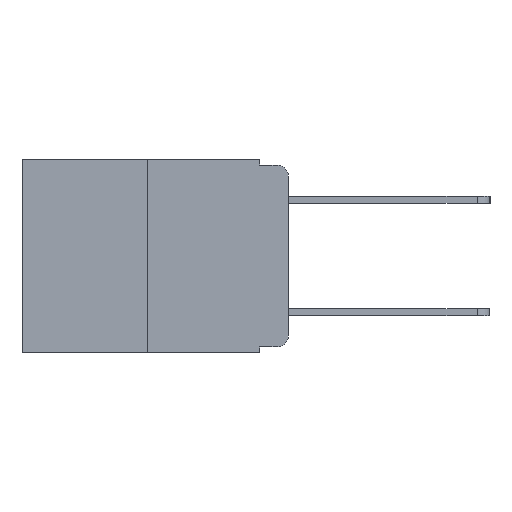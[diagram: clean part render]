
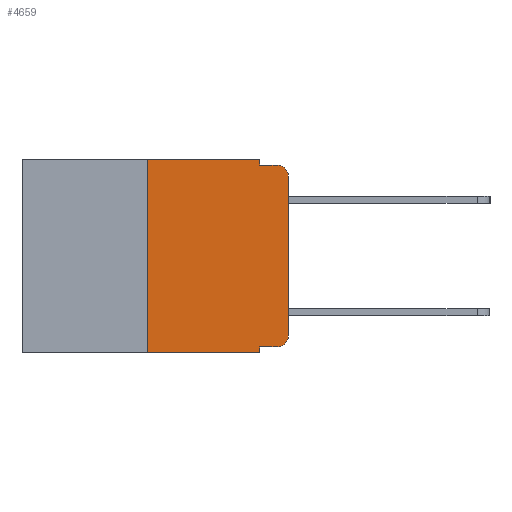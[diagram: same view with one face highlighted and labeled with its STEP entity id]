
A CAD part, left-side view. The second image highlights one B-rep face of the part: STEP entity #4659.
In plain terms, the highlighted planar face has unit normal (-1, 0, 0).
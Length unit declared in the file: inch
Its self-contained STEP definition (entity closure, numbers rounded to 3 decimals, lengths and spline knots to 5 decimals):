
#343 = DIRECTION ( 'NONE',  ( 0., 0., -1. ) ) ;
#415 = ORIENTED_EDGE ( 'NONE', *, *, #500, .T. ) ;
#500 = EDGE_CURVE ( 'NONE', #1813, #5621, #2623, .T. ) ;
#789 = LINE ( 'NONE', #902, #12038 ) ;
#824 = VERTEX_POINT ( 'NONE', #6479 ) ;
#839 = CARTESIAN_POINT ( 'NONE',  ( 0., 0.051, -0.343 ) ) ;
#902 = CARTESIAN_POINT ( 'NONE',  ( 0., 0.051, 0. ) ) ;
#933 = ORIENTED_EDGE ( 'NONE', *, *, #5554, .F. ) ;
#950 = VERTEX_POINT ( 'NONE', #839 ) ;
#1013 = VERTEX_POINT ( 'NONE', #8694 ) ;
#1298 = CARTESIAN_POINT ( 'NONE',  ( 0., 0.25, 0. ) ) ;
#1650 = VECTOR ( 'NONE', #11972, 39.37008 ) ;
#1764 = VERTEX_POINT ( 'NONE', #9532 ) ;
#1813 = VERTEX_POINT ( 'NONE', #7190 ) ;
#1817 = DIRECTION ( 'NONE',  ( 0., 0., -1. ) ) ;
#1917 = AXIS2_PLACEMENT_3D ( 'NONE', #5327, #12515, #6460 ) ;
#2474 = AXIS2_PLACEMENT_3D ( 'NONE', #7707, #5722, #5657 ) ;
#2623 = CIRCLE ( 'NONE', #3222, 0.02 ) ;
#2823 = CIRCLE ( 'NONE', #1917, 0.02 ) ;
#2984 = LINE ( 'NONE', #5390, #6049 ) ;
#3222 = AXIS2_PLACEMENT_3D ( 'NONE', #10448, #12787, #1817 ) ;
#3319 = VERTEX_POINT ( 'NONE', #11322 ) ;
#3447 = ORIENTED_EDGE ( 'NONE', *, *, #7054, .F. ) ;
#3523 = FACE_OUTER_BOUND ( 'NONE', #4366, .T. ) ;
#3734 = ORIENTED_EDGE ( 'NONE', *, *, #13476, .F. ) ;
#3756 = EDGE_CURVE ( 'NONE', #11343, #1813, #7503, .T. ) ;
#4064 = EDGE_CURVE ( 'NONE', #1013, #950, #789, .T. ) ;
#4366 = EDGE_LOOP ( 'NONE', ( #6656, #415, #3447, #933, #3734, #6722, #6639, #5891, #5738, #6790 ) ) ;
#4580 = CARTESIAN_POINT ( 'NONE',  ( 0., 0.473, -0.343 ) ) ;
#4587 = VECTOR ( 'NONE', #6284, 39.37008 ) ;
#4601 = DIRECTION ( 'NONE',  ( 0., -1., 0. ) ) ;
#4659 = ADVANCED_FACE ( 'NONE', ( #3523 ), #4942, .F. ) ;
#4846 = EDGE_CURVE ( 'NONE', #824, #12397, #6729, .T. ) ;
#4928 = EDGE_CURVE ( 'NONE', #824, #950, #10919, .T. ) ;
#4942 = PLANE ( 'NONE',  #2474 ) ;
#4946 = CARTESIAN_POINT ( 'NONE',  ( 0., 0., 0. ) ) ;
#5255 = CARTESIAN_POINT ( 'NONE',  ( 0., 0.02, -0.01 ) ) ;
#5327 = CARTESIAN_POINT ( 'NONE',  ( 0., 0.02, -0.313 ) ) ;
#5390 = CARTESIAN_POINT ( 'NONE',  ( 0., 0.051, -0.333 ) ) ;
#5554 = EDGE_CURVE ( 'NONE', #7035, #3319, #12079, .T. ) ;
#5621 = VERTEX_POINT ( 'NONE', #5255 ) ;
#5657 = DIRECTION ( 'NONE',  ( 0., 0., -1. ) ) ;
#5722 = DIRECTION ( 'NONE',  ( 1., 0., 0. ) ) ;
#5738 = ORIENTED_EDGE ( 'NONE', *, *, #13299, .T. ) ;
#5744 = CARTESIAN_POINT ( 'NONE',  ( 0., 0.051, 0. ) ) ;
#5773 = CARTESIAN_POINT ( 'NONE',  ( 0., 0.473, 0. ) ) ;
#5891 = ORIENTED_EDGE ( 'NONE', *, *, #4064, .F. ) ;
#6049 = VECTOR ( 'NONE', #11622, 39.37008 ) ;
#6055 = DIRECTION ( 'NONE',  ( 0., 0., 1. ) ) ;
#6284 = DIRECTION ( 'NONE',  ( 0., 0., 1. ) ) ;
#6460 = DIRECTION ( 'NONE',  ( 0., 0., -1. ) ) ;
#6479 = CARTESIAN_POINT ( 'NONE',  ( 0., 0.25, -0.343 ) ) ;
#6639 = ORIENTED_EDGE ( 'NONE', *, *, #4928, .T. ) ;
#6656 = ORIENTED_EDGE ( 'NONE', *, *, #3756, .T. ) ;
#6722 = ORIENTED_EDGE ( 'NONE', *, *, #4846, .F. ) ;
#6729 = LINE ( 'NONE', #9146, #12103 ) ;
#6790 = ORIENTED_EDGE ( 'NONE', *, *, #12036, .T. ) ;
#7035 = VERTEX_POINT ( 'NONE', #5744 ) ;
#7054 = EDGE_CURVE ( 'NONE', #3319, #5621, #10461, .T. ) ;
#7190 = CARTESIAN_POINT ( 'NONE',  ( 0., 0., -0.03 ) ) ;
#7503 = LINE ( 'NONE', #4946, #4587 ) ;
#7707 = CARTESIAN_POINT ( 'NONE',  ( 0., 0.473, 0. ) ) ;
#7772 = DIRECTION ( 'NONE',  ( 0., 0., -1. ) ) ;
#8441 = CARTESIAN_POINT ( 'NONE',  ( 0., 0.051, 0. ) ) ;
#8694 = CARTESIAN_POINT ( 'NONE',  ( 0., 0.051, -0.333 ) ) ;
#9082 = LINE ( 'NONE', #5773, #11381 ) ;
#9146 = CARTESIAN_POINT ( 'NONE',  ( 0., 0.25, 0. ) ) ;
#9532 = CARTESIAN_POINT ( 'NONE',  ( 0., 0.02, -0.333 ) ) ;
#9814 = VECTOR ( 'NONE', #343, 39.37008 ) ;
#10027 = CARTESIAN_POINT ( 'NONE',  ( 0., 0.051, -0.01 ) ) ;
#10448 = CARTESIAN_POINT ( 'NONE',  ( 0., 0.02, -0.03 ) ) ;
#10461 = LINE ( 'NONE', #10027, #1650 ) ;
#10919 = LINE ( 'NONE', #4580, #13128 ) ;
#11322 = CARTESIAN_POINT ( 'NONE',  ( 0., 0.051, -0.01 ) ) ;
#11343 = VERTEX_POINT ( 'NONE', #12303 ) ;
#11381 = VECTOR ( 'NONE', #13820, 39.37008 ) ;
#11622 = DIRECTION ( 'NONE',  ( 0., -1., 0. ) ) ;
#11972 = DIRECTION ( 'NONE',  ( 0., -1., 0. ) ) ;
#12036 = EDGE_CURVE ( 'NONE', #1764, #11343, #2823, .T. ) ;
#12038 = VECTOR ( 'NONE', #7772, 39.37008 ) ;
#12079 = LINE ( 'NONE', #8441, #9814 ) ;
#12103 = VECTOR ( 'NONE', #6055, 39.37008 ) ;
#12303 = CARTESIAN_POINT ( 'NONE',  ( 0., 0., -0.313 ) ) ;
#12397 = VERTEX_POINT ( 'NONE', #1298 ) ;
#12515 = DIRECTION ( 'NONE',  ( -1., 0., 0. ) ) ;
#12787 = DIRECTION ( 'NONE',  ( -1., 0., 0. ) ) ;
#13128 = VECTOR ( 'NONE', #4601, 39.37008 ) ;
#13299 = EDGE_CURVE ( 'NONE', #1013, #1764, #2984, .T. ) ;
#13476 = EDGE_CURVE ( 'NONE', #12397, #7035, #9082, .T. ) ;
#13820 = DIRECTION ( 'NONE',  ( 0., -1., 0. ) ) ;
